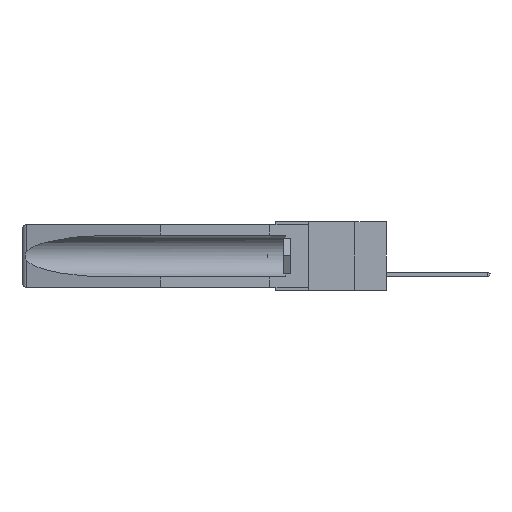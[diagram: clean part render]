
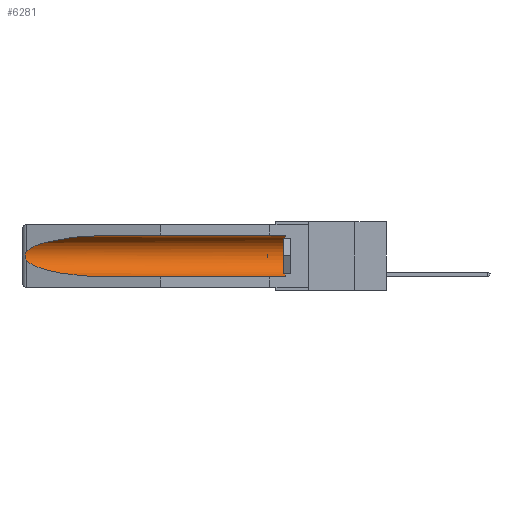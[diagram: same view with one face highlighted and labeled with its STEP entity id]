
A CAD part, left-side view. The second image highlights one B-rep face of the part: STEP entity #6281.
In plain terms, the highlighted cylindrical face has radius 2.857 mm (diameter 5.715 mm), a partial arc.
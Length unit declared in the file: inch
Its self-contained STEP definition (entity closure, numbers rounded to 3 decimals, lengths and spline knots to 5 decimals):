
#432 = CARTESIAN_POINT ( 'NONE',  ( 0.25451, 1.48313, -0.09465 ) ) ;
#477 = VERTEX_POINT ( 'NONE', #23048 ) ;
#600 = VERTEX_POINT ( 'NONE', #27706 ) ;
#3317 = DIRECTION ( 'NONE',  ( 0., 1., 0. ) ) ;
#3491 = LINE ( 'NONE', #14399, #30934 ) ;
#3688 =( BOUNDED_CURVE ( )  B_SPLINE_CURVE ( 3, ( #11178, #8904, #432, #13734 ),
 .UNSPECIFIED., .F., .F. ) 
 B_SPLINE_CURVE_WITH_KNOTS ( ( 4, 4 ),
 ( 4.71239, 6.08839 ),
 .UNSPECIFIED. ) 
 CURVE ( )  GEOMETRIC_REPRESENTATION_ITEM ( )  RATIONAL_B_SPLINE_CURVE ( ( 1., 0.848, 0.848, 1. ) ) 
 REPRESENTATION_ITEM ( '' )  );
#5104 = CARTESIAN_POINT ( 'NONE',  ( 0.2675, 1.53308, -0.17534 ) ) ;
#5336 = CARTESIAN_POINT ( 'NONE',  ( 0.26654, 1.53092, -0.15636 ) ) ;
#5411 = EDGE_LOOP ( 'NONE', ( #17118, #20659, #23292, #14278, #15948, #18259 ) ) ;
#6281 = ADVANCED_FACE ( 'NONE', ( #16129 ), #11208, .F. ) ;
#7213 = CARTESIAN_POINT ( 'NONE',  ( 0.155, 1.07973, -0.059 ) ) ;
#8140 = CARTESIAN_POINT ( 'NONE',  ( 0.21114, 1.30732, -0.284 ) ) ;
#8193 = VERTEX_POINT ( 'NONE', #32178 ) ;
#8426 = VERTEX_POINT ( 'NONE', #13808 ) ;
#8461 = DIRECTION ( 'NONE',  ( 0., 1., 0. ) ) ;
#8904 = CARTESIAN_POINT ( 'NONE',  ( 0.21114, 1.30732, -0.059 ) ) ;
#9287 = EDGE_CURVE ( 'NONE', #17147, #34264, #3688, .T. ) ;
#9656 = CARTESIAN_POINT ( 'NONE',  ( 0.26537, 1.52718, -0.14972 ) ) ;
#9820 = AXIS2_PLACEMENT_3D ( 'NONE', #27229, #24437, #32364 ) ;
#10790 = CARTESIAN_POINT ( 'NONE',  ( 0.25451, 1.48313, -0.24835 ) ) ;
#10980 = DIRECTION ( 'NONE',  ( 0., 0., 1. ) ) ;
#11178 = CARTESIAN_POINT ( 'NONE',  ( 0.155, 1.07973, -0.059 ) ) ;
#11208 = CYLINDRICAL_SURFACE ( 'NONE', #18516, 0.1125 ) ;
#12155 = EDGE_CURVE ( 'NONE', #34264, #477, #32011, .T. ) ;
#12783 = CARTESIAN_POINT ( 'NONE',  ( 0.2673, 1.53269, -0.17917 ) ) ;
#13734 = CARTESIAN_POINT ( 'NONE',  ( 0.26537, 1.52718, -0.14972 ) ) ;
#13808 = CARTESIAN_POINT ( 'NONE',  ( 0.155, 0.126, -0.059 ) ) ;
#14278 = ORIENTED_EDGE ( 'NONE', *, *, #16162, .F. ) ;
#14399 = CARTESIAN_POINT ( 'NONE',  ( 0.155, -0.30754, -0.059 ) ) ;
#15514 = CARTESIAN_POINT ( 'NONE',  ( 0.26597, 1.5296, -0.19026 ) ) ;
#15734 = CARTESIAN_POINT ( 'NONE',  ( 0.26597, 1.52961, -0.15275 ) ) ;
#15948 = ORIENTED_EDGE ( 'NONE', *, *, #24185, .T. ) ;
#16129 = FACE_OUTER_BOUND ( 'NONE', #5411, .T. ) ;
#16162 = EDGE_CURVE ( 'NONE', #8193, #600, #21702, .T. ) ;
#17118 = ORIENTED_EDGE ( 'NONE', *, *, #9287, .T. ) ;
#17147 = VERTEX_POINT ( 'NONE', #7213 ) ;
#18161 = CARTESIAN_POINT ( 'NONE',  ( 0.26537, 1.52718, -0.19328 ) ) ;
#18259 = ORIENTED_EDGE ( 'NONE', *, *, #23903, .T. ) ;
#18516 = AXIS2_PLACEMENT_3D ( 'NONE', #24348, #8461, #10980 ) ;
#19757 = EDGE_CURVE ( 'NONE', #477, #600, #33091, .T. ) ;
#20659 = ORIENTED_EDGE ( 'NONE', *, *, #12155, .T. ) ;
#20734 = CARTESIAN_POINT ( 'NONE',  ( 0.26537, 1.52718, -0.14972 ) ) ;
#21702 = LINE ( 'NONE', #32467, #22544 ) ;
#22544 = VECTOR ( 'NONE', #3317, 39.37008 ) ;
#23048 = CARTESIAN_POINT ( 'NONE',  ( 0.26537, 1.52718, -0.19328 ) ) ;
#23292 = ORIENTED_EDGE ( 'NONE', *, *, #19757, .T. ) ;
#23435 = CARTESIAN_POINT ( 'NONE',  ( 0.26655, 1.53094, -0.18657 ) ) ;
#23903 = EDGE_CURVE ( 'NONE', #8426, #17147, #3491, .T. ) ;
#24185 = EDGE_CURVE ( 'NONE', #8193, #8426, #30296, .T. ) ;
#24348 = CARTESIAN_POINT ( 'NONE',  ( 0.155, -0.30754, -0.1715 ) ) ;
#24437 = DIRECTION ( 'NONE',  ( 0., -1., 0. ) ) ;
#25296 = DIRECTION ( 'NONE',  ( 0., 1., 0. ) ) ;
#26476 = CARTESIAN_POINT ( 'NONE',  ( 0.26537, 1.52718, -0.19328 ) ) ;
#27229 = CARTESIAN_POINT ( 'NONE',  ( 0.155, 0.126, -0.1715 ) ) ;
#27706 = CARTESIAN_POINT ( 'NONE',  ( 0.155, 1.07973, -0.284 ) ) ;
#28702 = CARTESIAN_POINT ( 'NONE',  ( 0.2673, 1.5327, -0.16383 ) ) ;
#29053 = CARTESIAN_POINT ( 'NONE',  ( 0.155, 1.07973, -0.284 ) ) ;
#30296 = CIRCLE ( 'NONE', #9820, 0.1125 ) ;
#30934 = VECTOR ( 'NONE', #25296, 39.37008 ) ;
#31512 = CARTESIAN_POINT ( 'NONE',  ( 0.2675, 1.53308, -0.16763 ) ) ;
#32011 = B_SPLINE_CURVE_WITH_KNOTS ( 'NONE', 3,
 ( #20734, #15734, #5336, #28702, #31512, #5104, #12783, #23435, #15514, #18161 ),
 .UNSPECIFIED., .F., .F.,
 ( 4, 2, 2, 2, 4 ),
 ( 0., 0.00029, 0.00058, 0.00087, 0.00117 ),
 .UNSPECIFIED. ) ;
#32178 = CARTESIAN_POINT ( 'NONE',  ( 0.155, 0.126, -0.284 ) ) ;
#32364 = DIRECTION ( 'NONE',  ( 0., 0., 1. ) ) ;
#32467 = CARTESIAN_POINT ( 'NONE',  ( 0.155, -0.30754, -0.284 ) ) ;
#33091 =( BOUNDED_CURVE ( )  B_SPLINE_CURVE ( 3, ( #26476, #10790, #8140, #29053 ),
 .UNSPECIFIED., .F., .F. ) 
 B_SPLINE_CURVE_WITH_KNOTS ( ( 4, 4 ),
 ( 0.1948, 1.5708 ),
 .UNSPECIFIED. ) 
 CURVE ( )  GEOMETRIC_REPRESENTATION_ITEM ( )  RATIONAL_B_SPLINE_CURVE ( ( 1., 0.848, 0.848, 1. ) ) 
 REPRESENTATION_ITEM ( '' )  );
#34264 = VERTEX_POINT ( 'NONE', #9656 ) ;
